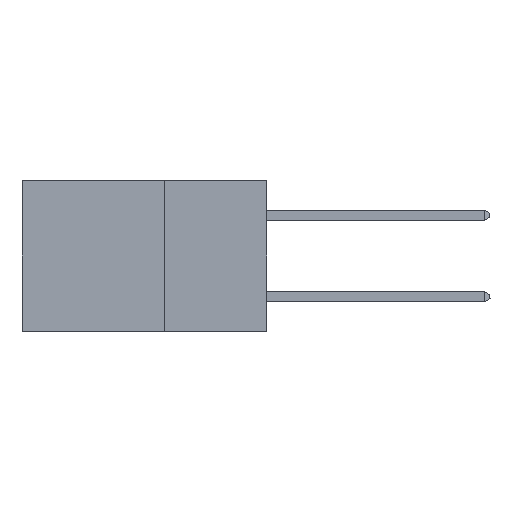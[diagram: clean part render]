
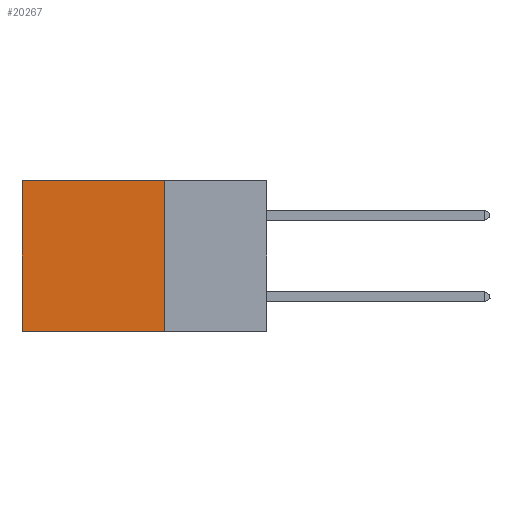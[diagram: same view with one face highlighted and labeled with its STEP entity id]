
A CAD part, left-side view. The second image highlights one B-rep face of the part: STEP entity #20267.
In plain terms, the highlighted planar face has unit normal (-1, 0, 0).
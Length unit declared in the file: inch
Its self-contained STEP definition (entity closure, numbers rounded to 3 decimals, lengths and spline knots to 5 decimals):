
#1141 = VECTOR ( 'NONE', #14553, 39.37008 ) ;
#1761 = DIRECTION ( 'NONE',  ( 0., 0., -1. ) ) ;
#3210 = VECTOR ( 'NONE', #1761, 39.37008 ) ;
#4918 = AXIS2_PLACEMENT_3D ( 'NONE', #9139, #28154, #12438 ) ;
#5473 = VERTEX_POINT ( 'NONE', #26118 ) ;
#8534 = LINE ( 'NONE', #39718, #1141 ) ;
#9139 = CARTESIAN_POINT ( 'NONE',  ( 0.2875, 0.25, 0. ) ) ;
#10185 = VECTOR ( 'NONE', #40793, 39.37008 ) ;
#10880 = EDGE_CURVE ( 'NONE', #5473, #29217, #8534, .T. ) ;
#12438 = DIRECTION ( 'NONE',  ( 0., 0., -1. ) ) ;
#14294 = CARTESIAN_POINT ( 'NONE',  ( 0.2875, 0.6, -0.37 ) ) ;
#14553 = DIRECTION ( 'NONE',  ( 0., 0., -1. ) ) ;
#14580 = CARTESIAN_POINT ( 'NONE',  ( 0.2875, 0.25, -0.37 ) ) ;
#15523 = EDGE_LOOP ( 'NONE', ( #27700, #24927, #17479, #21502 ) ) ;
#17479 = ORIENTED_EDGE ( 'NONE', *, *, #10880, .F. ) ;
#18773 = CARTESIAN_POINT ( 'NONE',  ( 0.2875, 0.25, -0.37 ) ) ;
#18831 = LINE ( 'NONE', #24632, #27199 ) ;
#18932 = EDGE_CURVE ( 'NONE', #5473, #34964, #18831, .T. ) ;
#20267 = ADVANCED_FACE ( 'NONE', ( #29642 ), #24725, .F. ) ;
#21068 = LINE ( 'NONE', #18773, #10185 ) ;
#21502 = ORIENTED_EDGE ( 'NONE', *, *, #18932, .T. ) ;
#24632 = CARTESIAN_POINT ( 'NONE',  ( 0.2875, 0.25, 0. ) ) ;
#24725 = PLANE ( 'NONE',  #4918 ) ;
#24927 = ORIENTED_EDGE ( 'NONE', *, *, #36970, .F. ) ;
#26118 = CARTESIAN_POINT ( 'NONE',  ( 0.2875, 0.25, 0. ) ) ;
#26846 = CARTESIAN_POINT ( 'NONE',  ( 0.2875, 0.6, 0. ) ) ;
#27199 = VECTOR ( 'NONE', #34275, 39.37008 ) ;
#27700 = ORIENTED_EDGE ( 'NONE', *, *, #37784, .T. ) ;
#28154 = DIRECTION ( 'NONE',  ( 1., 0., 0. ) ) ;
#29061 = VERTEX_POINT ( 'NONE', #14294 ) ;
#29217 = VERTEX_POINT ( 'NONE', #14580 ) ;
#29642 = FACE_OUTER_BOUND ( 'NONE', #15523, .T. ) ;
#30355 = LINE ( 'NONE', #26846, #3210 ) ;
#34275 = DIRECTION ( 'NONE',  ( 0., 1., 0. ) ) ;
#34826 = CARTESIAN_POINT ( 'NONE',  ( 0.2875, 0.6, 0. ) ) ;
#34964 = VERTEX_POINT ( 'NONE', #34826 ) ;
#36970 = EDGE_CURVE ( 'NONE', #29217, #29061, #21068, .T. ) ;
#37784 = EDGE_CURVE ( 'NONE', #34964, #29061, #30355, .T. ) ;
#39718 = CARTESIAN_POINT ( 'NONE',  ( 0.2875, 0.25, 0. ) ) ;
#40793 = DIRECTION ( 'NONE',  ( 0., 1., 0. ) ) ;
